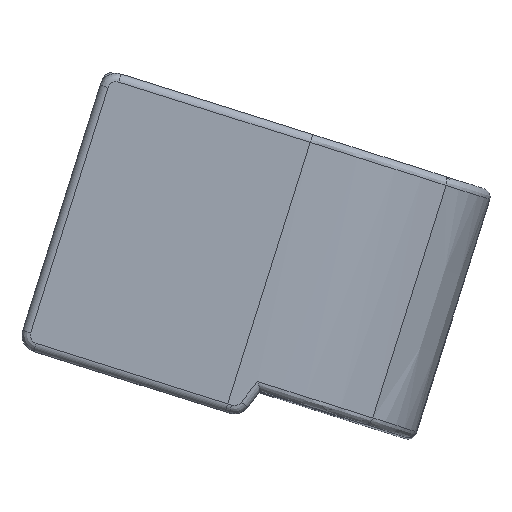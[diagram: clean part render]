
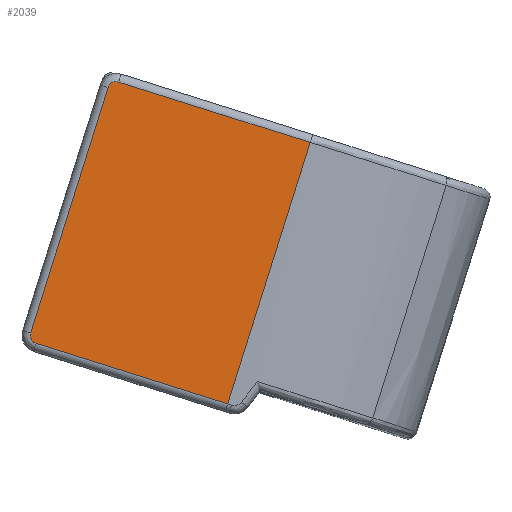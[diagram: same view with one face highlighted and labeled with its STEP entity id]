
A CAD part, top view. The second image highlights one B-rep face of the part: STEP entity #2039.
In plain terms, the highlighted planar face has unit normal (0, 0, 1).
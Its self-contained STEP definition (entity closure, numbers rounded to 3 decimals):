
#95=PLANE('',#2224);
#189=FACE_OUTER_BOUND('',#299,.T.);
#299=EDGE_LOOP('',(#1729,#1730,#1731,#1732,#1733,#1734));
#501=LINE('',#3547,#689);
#502=LINE('',#3566,#690);
#504=LINE('',#3586,#692);
#507=LINE('',#3737,#695);
#689=VECTOR('',#2671,10.);
#690=VECTOR('',#2682,10.);
#692=VECTOR('',#2694,10.);
#695=VECTOR('',#2713,10.);
#791=CIRCLE('',#2208,0.25);
#795=CIRCLE('',#2213,0.25);
#984=VERTEX_POINT('',#3537);
#985=VERTEX_POINT('',#3545);
#987=VERTEX_POINT('',#3558);
#989=VERTEX_POINT('',#3564);
#991=VERTEX_POINT('',#3578);
#993=VERTEX_POINT('',#3584);
#1258=EDGE_CURVE('',#985,#984,#501,.T.);
#1260=EDGE_CURVE('',#987,#985,#791,.T.);
#1263=EDGE_CURVE('',#989,#987,#502,.T.);
#1266=EDGE_CURVE('',#991,#989,#795,.T.);
#1269=EDGE_CURVE('',#993,#991,#504,.T.);
#1287=EDGE_CURVE('',#984,#993,#507,.T.);
#1729=ORIENTED_EDGE('',*,*,#1258,.F.);
#1730=ORIENTED_EDGE('',*,*,#1260,.F.);
#1731=ORIENTED_EDGE('',*,*,#1263,.F.);
#1732=ORIENTED_EDGE('',*,*,#1266,.F.);
#1733=ORIENTED_EDGE('',*,*,#1269,.F.);
#1734=ORIENTED_EDGE('',*,*,#1287,.F.);
#2039=ADVANCED_FACE('',(#189),#95,.T.);
#2208=AXIS2_PLACEMENT_3D('',#3560,#2674,#2675);
#2213=AXIS2_PLACEMENT_3D('',#3580,#2686,#2687);
#2224=AXIS2_PLACEMENT_3D('',#3736,#2711,#2712);
#2671=DIRECTION('',(0.954,-0.301,0.));
#2674=DIRECTION('center_axis',(0.,0.,
-1.));
#2675=DIRECTION('ref_axis',(-0.462,0.887,0.));
#2682=DIRECTION('',(0.301,0.954,0.));
#2686=DIRECTION('center_axis',(0.,0.,
-1.));
#2687=DIRECTION('ref_axis',(-0.887,-0.462,0.));
#2694=DIRECTION('',(-0.954,0.301,0.));
#2711=DIRECTION('center_axis',(0.,0.,
1.));
#2712=DIRECTION('ref_axis',(-0.954,0.301,0.));
#2713=DIRECTION('',(-0.301,-0.954,0.));
#3537=CARTESIAN_POINT('',(57.092,-31.746,14.433));
#3545=CARTESIAN_POINT('',(51.377,-29.944,14.433));
#3547=CARTESIAN_POINT('',(52.518,-30.303,14.433));
#3558=CARTESIAN_POINT('',(51.064,-30.107,14.433));
#3560=CARTESIAN_POINT('Origin',(51.302,-30.182,14.433));
#3564=CARTESIAN_POINT('',(48.756,-37.428,14.433));
#3566=CARTESIAN_POINT('',(51.312,-29.321,14.433));
#3578=CARTESIAN_POINT('',(48.919,-37.741,14.433));
#3580=CARTESIAN_POINT('Origin',(48.994,-37.503,14.433));
#3584=CARTESIAN_POINT('',(54.634,-39.543,14.433));
#3586=CARTESIAN_POINT('',(50.06,-38.101,14.433));
#3736=CARTESIAN_POINT('Origin',(57.265,-31.198,14.433));
#3737=CARTESIAN_POINT('',(57.265,-31.198,14.433));
